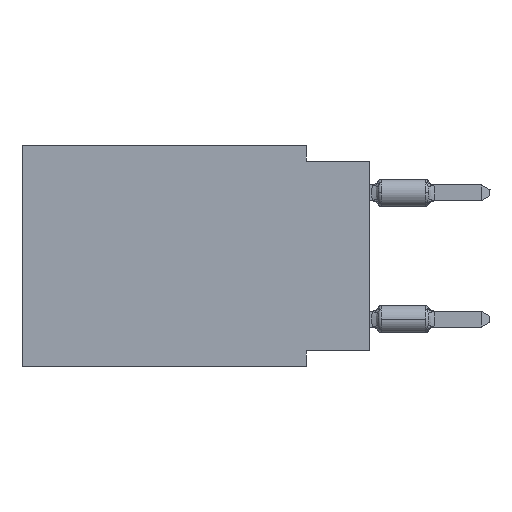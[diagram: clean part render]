
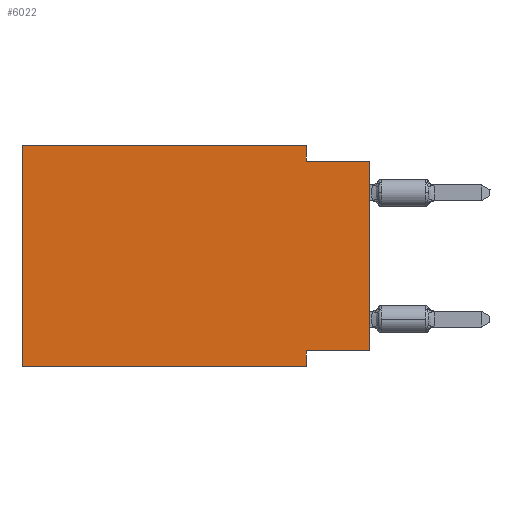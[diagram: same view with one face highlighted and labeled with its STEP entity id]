
A CAD part, left-side view. The second image highlights one B-rep face of the part: STEP entity #6022.
In plain terms, the highlighted planar face has unit normal (-1, 0, 0).
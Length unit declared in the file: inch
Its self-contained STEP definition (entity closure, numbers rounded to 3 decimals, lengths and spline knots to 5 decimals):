
#174 = VERTEX_POINT ( 'NONE', #7529 ) ;
#436 = EDGE_CURVE ( 'NONE', #24335, #174, #9575, .T. ) ;
#955 = DIRECTION ( 'NONE',  ( 0., 0., -1. ) ) ;
#1293 = CARTESIAN_POINT ( 'NONE',  ( 0., 0.55, 0. ) ) ;
#1520 = LINE ( 'NONE', #28287, #3652 ) ;
#1632 = CARTESIAN_POINT ( 'NONE',  ( 0., 0.1, 0. ) ) ;
#2923 = DIRECTION ( 'NONE',  ( 1., 0., 0. ) ) ;
#3652 = VECTOR ( 'NONE', #25706, 39.37008 ) ;
#3992 = LINE ( 'NONE', #30756, #15638 ) ;
#4158 = DIRECTION ( 'NONE',  ( 0., 0., 1. ) ) ;
#4540 = EDGE_CURVE ( 'NONE', #26355, #11564, #23347, .T. ) ;
#5216 = ORIENTED_EDGE ( 'NONE', *, *, #23714, .F. ) ;
#5451 = LINE ( 'NONE', #27835, #27530 ) ;
#5656 = CARTESIAN_POINT ( 'NONE',  ( 0., 0.55, 0. ) ) ;
#6003 = ORIENTED_EDGE ( 'NONE', *, *, #7725, .T. ) ;
#6022 = ADVANCED_FACE ( 'NONE', ( #10695 ), #10856, .F. ) ;
#6897 = EDGE_CURVE ( 'NONE', #26925, #174, #1520, .T. ) ;
#7352 = EDGE_CURVE ( 'NONE', #24335, #23146, #13934, .T. ) ;
#7529 = CARTESIAN_POINT ( 'NONE',  ( 0., 0.1, -0.35 ) ) ;
#7725 = EDGE_CURVE ( 'NONE', #29227, #28281, #3992, .T. ) ;
#8156 = LINE ( 'NONE', #15457, #24833 ) ;
#9332 = VECTOR ( 'NONE', #9720, 39.37008 ) ;
#9533 = ORIENTED_EDGE ( 'NONE', *, *, #12293, .F. ) ;
#9575 = LINE ( 'NONE', #24819, #9332 ) ;
#9720 = DIRECTION ( 'NONE',  ( 0., -1., 0. ) ) ;
#10416 = ORIENTED_EDGE ( 'NONE', *, *, #6897, .F. ) ;
#10695 = FACE_OUTER_BOUND ( 'NONE', #12986, .T. ) ;
#10856 = PLANE ( 'NONE',  #11927 ) ;
#10946 = DIRECTION ( 'NONE',  ( 0., -1., 0. ) ) ;
#11191 = DIRECTION ( 'NONE',  ( 0., 0., 1. ) ) ;
#11564 = VERTEX_POINT ( 'NONE', #15609 ) ;
#11927 = AXIS2_PLACEMENT_3D ( 'NONE', #5656, #2923, #955 ) ;
#12293 = EDGE_CURVE ( 'NONE', #11564, #28281, #22366, .T. ) ;
#12796 = CARTESIAN_POINT ( 'NONE',  ( 0., 0.1, 0. ) ) ;
#12986 = EDGE_LOOP ( 'NONE', ( #6003, #9533, #13454, #15692, #21033, #16321, #10416, #5216 ) ) ;
#13097 = CARTESIAN_POINT ( 'NONE',  ( 0., 0., -0.025 ) ) ;
#13454 = ORIENTED_EDGE ( 'NONE', *, *, #4540, .F. ) ;
#13934 = LINE ( 'NONE', #1293, #22887 ) ;
#15313 = CARTESIAN_POINT ( 'NONE',  ( 0., 0., -0.325 ) ) ;
#15457 = CARTESIAN_POINT ( 'NONE',  ( 0., 0.55, 0. ) ) ;
#15609 = CARTESIAN_POINT ( 'NONE',  ( 0., 0.1, -0.025 ) ) ;
#15638 = VECTOR ( 'NONE', #4158, 39.37008 ) ;
#15692 = ORIENTED_EDGE ( 'NONE', *, *, #29172, .F. ) ;
#15694 = DIRECTION ( 'NONE',  ( 0., 1., 0. ) ) ;
#15728 = DIRECTION ( 'NONE',  ( 0., 0., -1. ) ) ;
#16321 = ORIENTED_EDGE ( 'NONE', *, *, #436, .T. ) ;
#17627 = CARTESIAN_POINT ( 'NONE',  ( 0., 0.1, -0.325 ) ) ;
#17642 = VECTOR ( 'NONE', #10946, 39.37008 ) ;
#17755 = DIRECTION ( 'NONE',  ( 0., -1., 0. ) ) ;
#19185 = CARTESIAN_POINT ( 'NONE',  ( 0., 0.55, 0. ) ) ;
#20236 = CARTESIAN_POINT ( 'NONE',  ( 0., 0., -0.025 ) ) ;
#21033 = ORIENTED_EDGE ( 'NONE', *, *, #7352, .F. ) ;
#22366 = LINE ( 'NONE', #20236, #17642 ) ;
#22887 = VECTOR ( 'NONE', #11191, 39.37008 ) ;
#23146 = VERTEX_POINT ( 'NONE', #19185 ) ;
#23347 = LINE ( 'NONE', #12796, #27982 ) ;
#23714 = EDGE_CURVE ( 'NONE', #29227, #26925, #5451, .T. ) ;
#24335 = VERTEX_POINT ( 'NONE', #25859 ) ;
#24819 = CARTESIAN_POINT ( 'NONE',  ( 0., 0.55, -0.35 ) ) ;
#24833 = VECTOR ( 'NONE', #17755, 39.37008 ) ;
#25706 = DIRECTION ( 'NONE',  ( 0., 0., -1. ) ) ;
#25859 = CARTESIAN_POINT ( 'NONE',  ( 0., 0.55, -0.35 ) ) ;
#26355 = VERTEX_POINT ( 'NONE', #1632 ) ;
#26925 = VERTEX_POINT ( 'NONE', #17627 ) ;
#27530 = VECTOR ( 'NONE', #15694, 39.37008 ) ;
#27835 = CARTESIAN_POINT ( 'NONE',  ( 0., 0., -0.325 ) ) ;
#27982 = VECTOR ( 'NONE', #15728, 39.37008 ) ;
#28281 = VERTEX_POINT ( 'NONE', #13097 ) ;
#28287 = CARTESIAN_POINT ( 'NONE',  ( 0., 0.1, -0.35 ) ) ;
#29172 = EDGE_CURVE ( 'NONE', #23146, #26355, #8156, .T. ) ;
#29227 = VERTEX_POINT ( 'NONE', #15313 ) ;
#30756 = CARTESIAN_POINT ( 'NONE',  ( 0., 0., 0. ) ) ;
